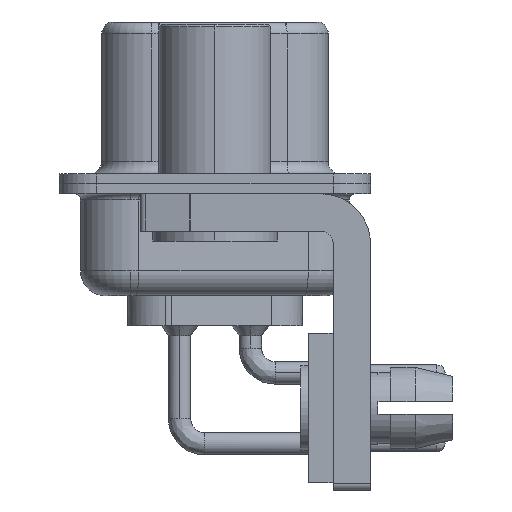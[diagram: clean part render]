
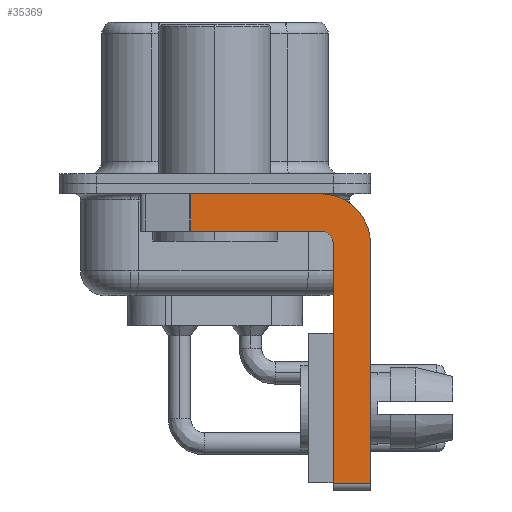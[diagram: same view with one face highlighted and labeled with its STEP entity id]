
A CAD part, left-side view. The second image highlights one B-rep face of the part: STEP entity #35369.
In plain terms, the highlighted planar face has unit normal (-1, 0, 0).
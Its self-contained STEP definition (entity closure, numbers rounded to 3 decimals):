
#272 = DIRECTION ( 'NONE',  ( 0., -1., 0. ) ) ;
#553 = VECTOR ( 'NONE', #4807, 1000. ) ;
#615 = EDGE_CURVE ( 'NONE', #29232, #36854, #22836, .T. ) ;
#890 = ORIENTED_EDGE ( 'NONE', *, *, #13170, .F. ) ;
#960 = DIRECTION ( 'NONE',  ( 0., 0., -1. ) ) ;
#1652 = VERTEX_POINT ( 'NONE', #31683 ) ;
#2175 = DIRECTION ( 'NONE',  ( 0., -1., 0. ) ) ;
#2203 = ORIENTED_EDGE ( 'NONE', *, *, #22692, .F. ) ;
#2740 = DIRECTION ( 'NONE',  ( 0., 0., -1. ) ) ;
#3222 = ORIENTED_EDGE ( 'NONE', *, *, #28864, .F. ) ;
#3931 = VERTEX_POINT ( 'NONE', #32968 ) ;
#4807 = DIRECTION ( 'NONE',  ( 0., 0., 1. ) ) ;
#4854 = CARTESIAN_POINT ( 'NONE',  ( -2.9, -4.25, -2.4 ) ) ;
#5306 = CARTESIAN_POINT ( 'NONE',  ( -2.9, 0.978, -0.4 ) ) ;
#7254 = VECTOR ( 'NONE', #19565, 1000. ) ;
#7724 = CARTESIAN_POINT ( 'NONE',  ( -2.9, -4.75, -12.3 ) ) ;
#7781 = DIRECTION ( 'NONE',  ( 0., 0., 1. ) ) ;
#8212 = LINE ( 'NONE', #7724, #553 ) ;
#8905 = AXIS2_PLACEMENT_3D ( 'NONE', #35100, #18091, #960 ) ;
#11053 = AXIS2_PLACEMENT_3D ( 'NONE', #17018, #28293, #2740 ) ;
#11861 = EDGE_CURVE ( 'NONE', #23133, #19959, #30891, .T. ) ;
#12630 = CARTESIAN_POINT ( 'NONE',  ( -2.9, 0.978, -1.9 ) ) ;
#12994 = VERTEX_POINT ( 'NONE', #32521 ) ;
#13170 = EDGE_CURVE ( 'NONE', #16944, #3931, #17060, .T. ) ;
#13556 = CARTESIAN_POINT ( 'NONE',  ( -2.9, -4.25, -1.9 ) ) ;
#13889 = CARTESIAN_POINT ( 'NONE',  ( -2.9, -6.25, -2.4 ) ) ;
#14255 = CARTESIAN_POINT ( 'NONE',  ( -2.9, -4.75, -2.4 ) ) ;
#14927 = CARTESIAN_POINT ( 'NONE',  ( -2.9, 3., -0.4 ) ) ;
#15083 = LINE ( 'NONE', #13556, #30141 ) ;
#16944 = VERTEX_POINT ( 'NONE', #14255 ) ;
#17018 = CARTESIAN_POINT ( 'NONE',  ( -2.9, -4.25, -2.4 ) ) ;
#17060 = CIRCLE ( 'NONE', #23396, 0.5 ) ;
#17653 = ORIENTED_EDGE ( 'NONE', *, *, #30450, .T. ) ;
#17780 = VECTOR ( 'NONE', #29565, 1000. ) ;
#18091 = DIRECTION ( 'NONE',  ( 1., 0., 0. ) ) ;
#18232 = CARTESIAN_POINT ( 'NONE',  ( -2.9, -4.75, -12.05 ) ) ;
#18436 = CARTESIAN_POINT ( 'NONE',  ( -2.9, -6.25, -12.05 ) ) ;
#18591 = CARTESIAN_POINT ( 'NONE',  ( -2.9, -4.25, -0.4 ) ) ;
#18664 = LINE ( 'NONE', #12630, #17780 ) ;
#19565 = DIRECTION ( 'NONE',  ( 0., 0., -1. ) ) ;
#19866 = PLANE ( 'NONE',  #11053 ) ;
#19959 = VERTEX_POINT ( 'NONE', #18436 ) ;
#21073 = VECTOR ( 'NONE', #272, 1000. ) ;
#21226 = ORIENTED_EDGE ( 'NONE', *, *, #11861, .T. ) ;
#21535 = ORIENTED_EDGE ( 'NONE', *, *, #27000, .F. ) ;
#22394 = LINE ( 'NONE', #13889, #7254 ) ;
#22692 = EDGE_CURVE ( 'NONE', #3931, #12994, #15083, .T. ) ;
#22836 = LINE ( 'NONE', #14927, #21073 ) ;
#23133 = VERTEX_POINT ( 'NONE', #18232 ) ;
#23360 = VECTOR ( 'NONE', #2175, 1000. ) ;
#23396 = AXIS2_PLACEMENT_3D ( 'NONE', #4854, #24826, #7781 ) ;
#24826 = DIRECTION ( 'NONE',  ( -1., 0., 0. ) ) ;
#25067 = ORIENTED_EDGE ( 'NONE', *, *, #27509, .F. ) ;
#27000 = EDGE_CURVE ( 'NONE', #1652, #19959, #22394, .T. ) ;
#27509 = EDGE_CURVE ( 'NONE', #23133, #16944, #8212, .T. ) ;
#28293 = DIRECTION ( 'NONE',  ( 1., 0., 0. ) ) ;
#28864 = EDGE_CURVE ( 'NONE', #36854, #1652, #34766, .T. ) ;
#29232 = VERTEX_POINT ( 'NONE', #5306 ) ;
#29565 = DIRECTION ( 'NONE',  ( 0., 0., -1. ) ) ;
#30027 = ORIENTED_EDGE ( 'NONE', *, *, #615, .F. ) ;
#30141 = VECTOR ( 'NONE', #33408, 1000. ) ;
#30450 = EDGE_CURVE ( 'NONE', #29232, #12994, #18664, .T. ) ;
#30891 = LINE ( 'NONE', #33352, #23360 ) ;
#31683 = CARTESIAN_POINT ( 'NONE',  ( -2.9, -6.25, -2.4 ) ) ;
#31808 = EDGE_LOOP ( 'NONE', ( #30027, #17653, #2203, #890, #25067, #21226, #21535, #3222 ) ) ;
#32319 = FACE_OUTER_BOUND ( 'NONE', #31808, .T. ) ;
#32521 = CARTESIAN_POINT ( 'NONE',  ( -2.9, 0.978, -1.9 ) ) ;
#32968 = CARTESIAN_POINT ( 'NONE',  ( -2.9, -4.25, -1.9 ) ) ;
#33352 = CARTESIAN_POINT ( 'NONE',  ( -2.9, -4.25, -12.05 ) ) ;
#33408 = DIRECTION ( 'NONE',  ( 0., 1., 0. ) ) ;
#34766 = CIRCLE ( 'NONE', #8905, 2. ) ;
#35100 = CARTESIAN_POINT ( 'NONE',  ( -2.9, -4.25, -2.4 ) ) ;
#35369 = ADVANCED_FACE ( 'NONE', ( #32319 ), #19866, .F. ) ;
#36854 = VERTEX_POINT ( 'NONE', #18591 ) ;
